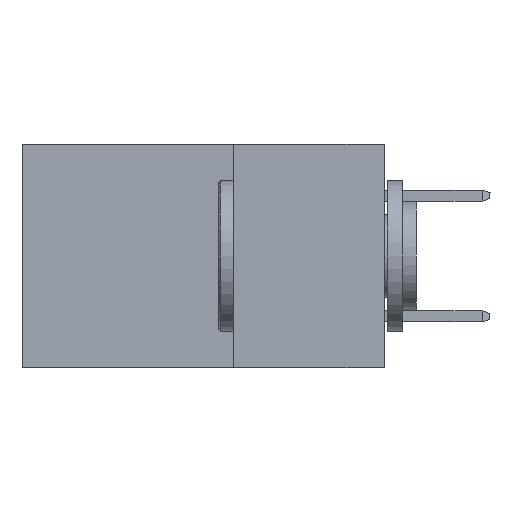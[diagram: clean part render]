
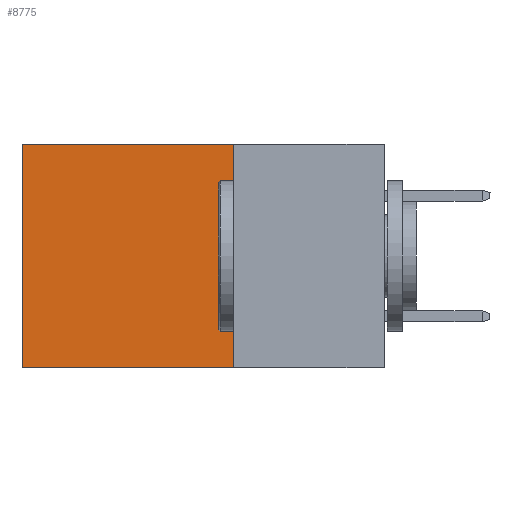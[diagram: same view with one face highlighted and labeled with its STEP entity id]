
A CAD part, left-side view. The second image highlights one B-rep face of the part: STEP entity #8775.
In plain terms, the highlighted planar face has unit normal (-1, 0, 0).
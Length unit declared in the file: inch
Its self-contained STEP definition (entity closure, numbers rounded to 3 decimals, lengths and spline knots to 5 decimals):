
#196 = EDGE_CURVE ( 'NONE', #5774, #30875, #4641, .T. ) ;
#1215 = CARTESIAN_POINT ( 'NONE',  ( 0.298, 0.6, 0. ) ) ;
#1688 = ORIENTED_EDGE ( 'NONE', *, *, #7311, .F. ) ;
#2545 = EDGE_LOOP ( 'NONE', ( #18846, #1688, #3802, #33786 ) ) ;
#3711 = VERTEX_POINT ( 'NONE', #26519 ) ;
#3802 = ORIENTED_EDGE ( 'NONE', *, *, #18626, .F. ) ;
#4641 = LINE ( 'NONE', #24928, #10370 ) ;
#4945 = VECTOR ( 'NONE', #27276, 39.37008 ) ;
#5058 = DIRECTION ( 'NONE',  ( 1., 0., 0. ) ) ;
#5774 = VERTEX_POINT ( 'NONE', #33271 ) ;
#6381 = CARTESIAN_POINT ( 'NONE',  ( 0.298, 0.25, -0.37 ) ) ;
#7246 = CARTESIAN_POINT ( 'NONE',  ( 0.298, 0.25, 0. ) ) ;
#7311 = EDGE_CURVE ( 'NONE', #9109, #3711, #18820, .T. ) ;
#8469 = VECTOR ( 'NONE', #30948, 39.37008 ) ;
#8775 = ADVANCED_FACE ( 'NONE', ( #29447 ), #33349, .F. ) ;
#9109 = VERTEX_POINT ( 'NONE', #6381 ) ;
#10370 = VECTOR ( 'NONE', #32833, 39.37008 ) ;
#11574 = CARTESIAN_POINT ( 'NONE',  ( 0.298, 0.25, -0.37 ) ) ;
#12371 = EDGE_CURVE ( 'NONE', #30875, #3711, #12777, .T. ) ;
#12777 = LINE ( 'NONE', #1215, #25905 ) ;
#17505 = CARTESIAN_POINT ( 'NONE',  ( 0.298, 0.6, 0. ) ) ;
#17592 = DIRECTION ( 'NONE',  ( 0., 0., -1. ) ) ;
#18626 = EDGE_CURVE ( 'NONE', #5774, #9109, #33017, .T. ) ;
#18820 = LINE ( 'NONE', #11574, #4945 ) ;
#18846 = ORIENTED_EDGE ( 'NONE', *, *, #12371, .T. ) ;
#19492 = DIRECTION ( 'NONE',  ( 0., 0., -1. ) ) ;
#24928 = CARTESIAN_POINT ( 'NONE',  ( 0.298, 0.25, 0. ) ) ;
#25869 = CARTESIAN_POINT ( 'NONE',  ( 0.298, 0.25, 0. ) ) ;
#25905 = VECTOR ( 'NONE', #19492, 39.37008 ) ;
#26519 = CARTESIAN_POINT ( 'NONE',  ( 0.298, 0.6, -0.37 ) ) ;
#27276 = DIRECTION ( 'NONE',  ( 0., 1., 0. ) ) ;
#29447 = FACE_OUTER_BOUND ( 'NONE', #2545, .T. ) ;
#30875 = VERTEX_POINT ( 'NONE', #17505 ) ;
#30948 = DIRECTION ( 'NONE',  ( 0., 0., -1. ) ) ;
#32833 = DIRECTION ( 'NONE',  ( 0., 1., 0. ) ) ;
#33017 = LINE ( 'NONE', #7246, #8469 ) ;
#33271 = CARTESIAN_POINT ( 'NONE',  ( 0.298, 0.25, 0. ) ) ;
#33349 = PLANE ( 'NONE',  #33579 ) ;
#33579 = AXIS2_PLACEMENT_3D ( 'NONE', #25869, #5058, #17592 ) ;
#33786 = ORIENTED_EDGE ( 'NONE', *, *, #196, .T. ) ;
